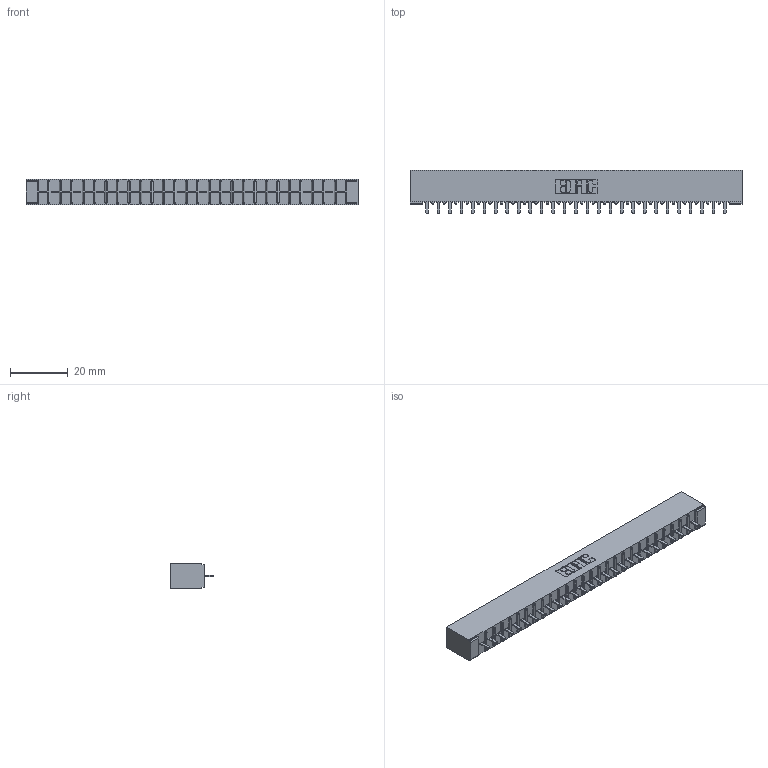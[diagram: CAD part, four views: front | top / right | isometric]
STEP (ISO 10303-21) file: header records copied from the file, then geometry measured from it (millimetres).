
FILE_DESCRIPTION (( 'STEP AP203' ), '1' );
FILE_NAME ('316-027-521-101.STEP', '2018-07-31T02:47:18', ( '' ), ( '' ), 'SwSTEP 2.0', 'SolidWorks 2016', '' );
FILE_SCHEMA (( 'CONFIG_CONTROL_DESIGN' ));
Length unit declared in the file: inch
Products named in the file (3): 306 Part_No Mounting; 306-290-001_121; 316-027-521-101
Assembly tree (28 placements, depth 2):
  316-027-521-101
    306 Part_No Mounting
    306-290-001_121  x27
Bounding box: 114.86 x 14.88 x 8.71 mm (x, y, z)
Volume: 8123.4 mm3; surface area: 12229.6 mm2
Topology: 28 solids, 28 shells, 1998 faces, 5611 edges, 3594 vertices
Faces by surface type: plane 1333, cylinder 557, sphere 108
Entity records: 26800 total; most frequent: CARTESIAN_POINT 4496, ORIENTED_EDGE 4454, DIRECTION 4435, EDGE_CURVE 2227, VECTOR 1737, LINE 1737, VERTEX_POINT 1410, AXIS2_PLACEMENT_3D 1349
